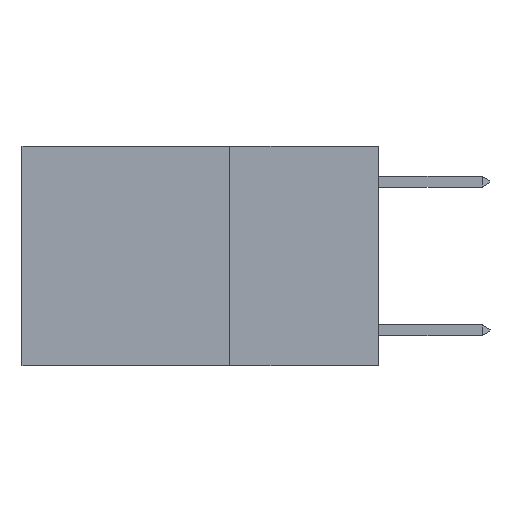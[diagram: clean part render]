
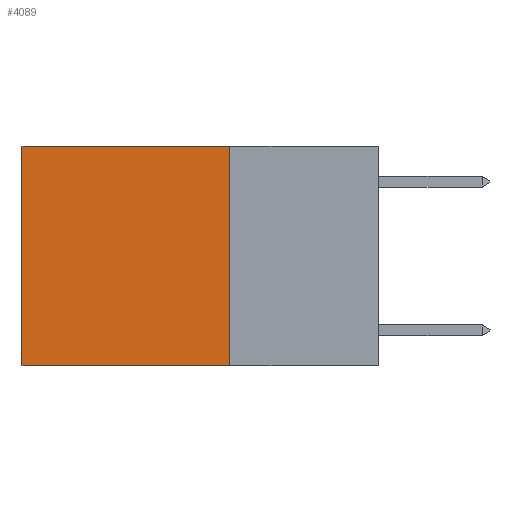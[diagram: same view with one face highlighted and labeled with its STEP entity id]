
A CAD part, left-side view. The second image highlights one B-rep face of the part: STEP entity #4089.
In plain terms, the highlighted planar face has unit normal (-1, 0, 0).
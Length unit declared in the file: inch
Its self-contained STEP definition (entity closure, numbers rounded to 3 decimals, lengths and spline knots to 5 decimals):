
#67 = LINE ( 'NONE', #1134, #6925 ) ;
#170 = DIRECTION ( 'NONE',  ( 0., 0., -1. ) ) ;
#1134 = CARTESIAN_POINT ( 'NONE',  ( 0.2625, 0.25, 0. ) ) ;
#1189 = LINE ( 'NONE', #8410, #3300 ) ;
#1396 = VERTEX_POINT ( 'NONE', #2686 ) ;
#1455 = VERTEX_POINT ( 'NONE', #1837 ) ;
#1587 = EDGE_CURVE ( 'NONE', #1396, #10757, #67, .T. ) ;
#1837 = CARTESIAN_POINT ( 'NONE',  ( 0.2625, 0.6, 0. ) ) ;
#2345 = CARTESIAN_POINT ( 'NONE',  ( 0.2625, 0.25, 0. ) ) ;
#2372 = CARTESIAN_POINT ( 'NONE',  ( 0.2625, 0.6, 0. ) ) ;
#2686 = CARTESIAN_POINT ( 'NONE',  ( 0.2625, 0.25, 0. ) ) ;
#3050 = VERTEX_POINT ( 'NONE', #5951 ) ;
#3270 = DIRECTION ( 'NONE',  ( 0., 0., -1. ) ) ;
#3300 = VECTOR ( 'NONE', #3364, 39.37008 ) ;
#3364 = DIRECTION ( 'NONE',  ( 0., 1., 0. ) ) ;
#3720 = CARTESIAN_POINT ( 'NONE',  ( 0.2625, 0.25, -0.37 ) ) ;
#3823 = EDGE_CURVE ( 'NONE', #1396, #1455, #1189, .T. ) ;
#3987 = ORIENTED_EDGE ( 'NONE', *, *, #3823, .T. ) ;
#3993 = LINE ( 'NONE', #3720, #8143 ) ;
#4089 = ADVANCED_FACE ( 'NONE', ( #10151 ), #5989, .F. ) ;
#4689 = DIRECTION ( 'NONE',  ( 0., 1., 0. ) ) ;
#5236 = EDGE_CURVE ( 'NONE', #10757, #3050, #3993, .T. ) ;
#5951 = CARTESIAN_POINT ( 'NONE',  ( 0.2625, 0.6, -0.37 ) ) ;
#5989 = PLANE ( 'NONE',  #8135 ) ;
#6925 = VECTOR ( 'NONE', #170, 39.37008 ) ;
#7647 = ORIENTED_EDGE ( 'NONE', *, *, #1587, .F. ) ;
#8037 = ORIENTED_EDGE ( 'NONE', *, *, #8400, .T. ) ;
#8135 = AXIS2_PLACEMENT_3D ( 'NONE', #2345, #8322, #3270 ) ;
#8143 = VECTOR ( 'NONE', #4689, 39.37008 ) ;
#8322 = DIRECTION ( 'NONE',  ( 1., 0., 0. ) ) ;
#8344 = DIRECTION ( 'NONE',  ( 0., 0., -1. ) ) ;
#8400 = EDGE_CURVE ( 'NONE', #1455, #3050, #8723, .T. ) ;
#8410 = CARTESIAN_POINT ( 'NONE',  ( 0.2625, 0.25, 0. ) ) ;
#8723 = LINE ( 'NONE', #2372, #9194 ) ;
#8856 = CARTESIAN_POINT ( 'NONE',  ( 0.2625, 0.25, -0.37 ) ) ;
#9067 = ORIENTED_EDGE ( 'NONE', *, *, #5236, .F. ) ;
#9194 = VECTOR ( 'NONE', #8344, 39.37008 ) ;
#9592 = EDGE_LOOP ( 'NONE', ( #8037, #9067, #7647, #3987 ) ) ;
#10151 = FACE_OUTER_BOUND ( 'NONE', #9592, .T. ) ;
#10757 = VERTEX_POINT ( 'NONE', #8856 ) ;
